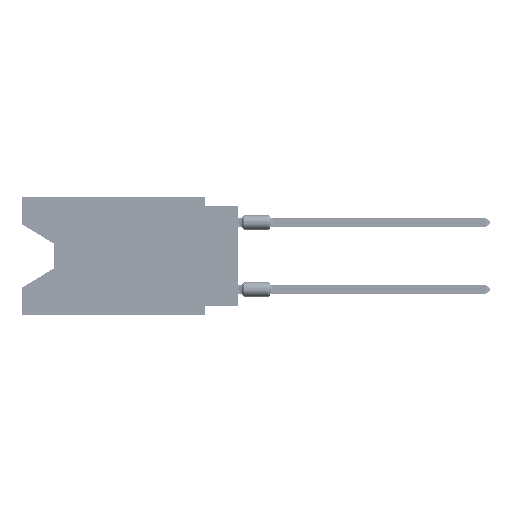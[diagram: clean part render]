
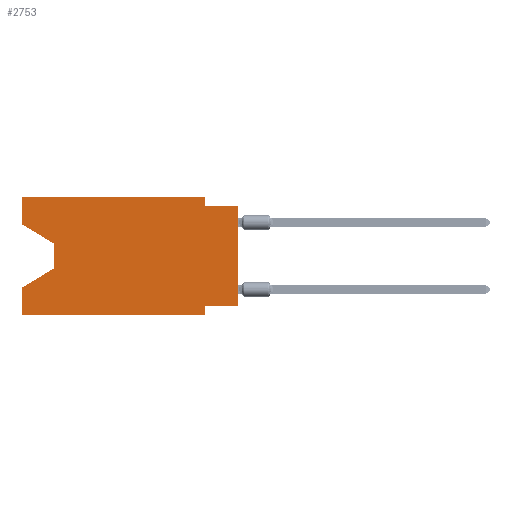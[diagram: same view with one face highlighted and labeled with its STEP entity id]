
A CAD part, left-side view. The second image highlights one B-rep face of the part: STEP entity #2753.
In plain terms, the highlighted planar face has unit normal (-1, 0, 0).
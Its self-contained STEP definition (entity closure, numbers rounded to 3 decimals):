
#519 = LINE ( 'NONE', #11945, #1159 ) ;
#1133 = VERTEX_POINT ( 'NONE', #64402 ) ;
#1159 = VECTOR ( 'NONE', #6578, 1000. ) ;
#1342 = CARTESIAN_POINT ( 'NONE',  ( 0., 2.54, -8.89 ) ) ;
#1442 = CARTESIAN_POINT ( 'NONE',  ( 0., 16.383, -2.038 ) ) ;
#2239 = CARTESIAN_POINT ( 'NONE',  ( 0., 0., -8.255 ) ) ;
#2268 = ORIENTED_EDGE ( 'NONE', *, *, #3347, .T. ) ;
#2678 = CARTESIAN_POINT ( 'NONE',  ( 0., 2.54, 0. ) ) ;
#2753 = ADVANCED_FACE ( 'NONE', ( #69702 ), #36085, .F. ) ;
#3181 = CARTESIAN_POINT ( 'NONE',  ( 0., 2.54, 0. ) ) ;
#3347 = EDGE_CURVE ( 'NONE', #59369, #17152, #27628, .T. ) ;
#3630 = VERTEX_POINT ( 'NONE', #37940 ) ;
#3878 = CARTESIAN_POINT ( 'NONE',  ( 0., 16.383, 0. ) ) ;
#5182 = LINE ( 'NONE', #21991, #12365 ) ;
#5414 = EDGE_CURVE ( 'NONE', #59369, #1133, #24259, .T. ) ;
#6153 = CARTESIAN_POINT ( 'NONE',  ( 0., 0., 0. ) ) ;
#6578 = DIRECTION ( 'NONE',  ( 0., 0., 1. ) ) ;
#7423 = EDGE_CURVE ( 'NONE', #66414, #23507, #519, .T. ) ;
#8604 = ORIENTED_EDGE ( 'NONE', *, *, #28505, .F. ) ;
#8890 = VECTOR ( 'NONE', #50507, 1000. ) ;
#11186 = VERTEX_POINT ( 'NONE', #29836 ) ;
#11945 = CARTESIAN_POINT ( 'NONE',  ( 0., 16.383, 0. ) ) ;
#12365 = VECTOR ( 'NONE', #44164, 1000. ) ;
#13409 = DIRECTION ( 'NONE',  ( 0., 0., -1. ) ) ;
#13737 = CARTESIAN_POINT ( 'NONE',  ( 0., 16.383, 0. ) ) ;
#13738 = CARTESIAN_POINT ( 'NONE',  ( 0., 16.383, -8.89 ) ) ;
#14164 = LINE ( 'NONE', #68916, #43706 ) ;
#15554 = VERTEX_POINT ( 'NONE', #50233 ) ;
#17152 = VERTEX_POINT ( 'NONE', #18348 ) ;
#17781 = DIRECTION ( 'NONE',  ( 0., 0., -1. ) ) ;
#18108 = ORIENTED_EDGE ( 'NONE', *, *, #29094, .F. ) ;
#18138 = LINE ( 'NONE', #1342, #26150 ) ;
#18348 = CARTESIAN_POINT ( 'NONE',  ( 0., 0., -0.635 ) ) ;
#18890 = CARTESIAN_POINT ( 'NONE',  ( 0., 0., -8.255 ) ) ;
#19548 = ORIENTED_EDGE ( 'NONE', *, *, #32908, .F. ) ;
#20295 = DIRECTION ( 'NONE',  ( 0., 0., -1. ) ) ;
#20742 = ORIENTED_EDGE ( 'NONE', *, *, #32326, .T. ) ;
#21483 = CARTESIAN_POINT ( 'NONE',  ( 0., 13.97, -5.385 ) ) ;
#21991 = CARTESIAN_POINT ( 'NONE',  ( 0., 0., -0.635 ) ) ;
#23507 = VERTEX_POINT ( 'NONE', #62179 ) ;
#23662 = EDGE_CURVE ( 'NONE', #39236, #63906, #57859, .T. ) ;
#24259 = LINE ( 'NONE', #18890, #60516 ) ;
#25183 = ORIENTED_EDGE ( 'NONE', *, *, #33710, .T. ) ;
#25686 = DIRECTION ( 'NONE',  ( 1., 0., 0. ) ) ;
#26150 = VECTOR ( 'NONE', #17781, 1000. ) ;
#26580 = ORIENTED_EDGE ( 'NONE', *, *, #63363, .T. ) ;
#26687 = ORIENTED_EDGE ( 'NONE', *, *, #5414, .F. ) ;
#27628 = LINE ( 'NONE', #6153, #8890 ) ;
#28505 = EDGE_CURVE ( 'NONE', #11186, #17152, #5182, .T. ) ;
#29094 = EDGE_CURVE ( 'NONE', #1133, #15554, #18138, .T. ) ;
#29836 = CARTESIAN_POINT ( 'NONE',  ( 0., 2.54, -0.635 ) ) ;
#32326 = EDGE_CURVE ( 'NONE', #63906, #23507, #66678, .T. ) ;
#32908 = EDGE_CURVE ( 'NONE', #65284, #11186, #51334, .T. ) ;
#33710 = EDGE_CURVE ( 'NONE', #46148, #39236, #67631, .T. ) ;
#35056 = CARTESIAN_POINT ( 'NONE',  ( 0., 16.383, -8.89 ) ) ;
#36085 = PLANE ( 'NONE',  #37398 ) ;
#37108 = CARTESIAN_POINT ( 'NONE',  ( 0., 13.97, -3.505 ) ) ;
#37398 = AXIS2_PLACEMENT_3D ( 'NONE', #3878, #25686, #47519 ) ;
#37940 = CARTESIAN_POINT ( 'NONE',  ( 0., 16.383, 0. ) ) ;
#38931 = ORIENTED_EDGE ( 'NONE', *, *, #56579, .F. ) ;
#39006 = DIRECTION ( 'NONE',  ( 0., -0.855, -0.519 ) ) ;
#39021 = VECTOR ( 'NONE', #61651, 1000. ) ;
#39236 = VERTEX_POINT ( 'NONE', #61716 ) ;
#39835 = CARTESIAN_POINT ( 'NONE',  ( 0., 13.97, -5.385 ) ) ;
#40435 = VECTOR ( 'NONE', #58782, 1000. ) ;
#41642 = LINE ( 'NONE', #13738, #40435 ) ;
#41718 = DIRECTION ( 'NONE',  ( 0., 0., 1. ) ) ;
#42177 = VECTOR ( 'NONE', #62758, 1000. ) ;
#43444 = CARTESIAN_POINT ( 'NONE',  ( 0., 16.383, -2.038 ) ) ;
#43706 = VECTOR ( 'NONE', #41718, 1000. ) ;
#44164 = DIRECTION ( 'NONE',  ( 0., -1., 0. ) ) ;
#46148 = VERTEX_POINT ( 'NONE', #43444 ) ;
#47519 = DIRECTION ( 'NONE',  ( 0., 0., -1. ) ) ;
#48758 = ORIENTED_EDGE ( 'NONE', *, *, #7423, .F. ) ;
#50233 = CARTESIAN_POINT ( 'NONE',  ( 0., 2.54, -8.89 ) ) ;
#50507 = DIRECTION ( 'NONE',  ( 0., 0., 1. ) ) ;
#51334 = LINE ( 'NONE', #2678, #59666 ) ;
#54314 = EDGE_LOOP ( 'NONE', ( #25183, #67473, #20742, #48758, #26580, #18108, #26687, #2268, #8604, #19548, #38931, #62961 ) ) ;
#56579 = EDGE_CURVE ( 'NONE', #3630, #65284, #57383, .T. ) ;
#57383 = LINE ( 'NONE', #13737, #42177 ) ;
#57514 = DIRECTION ( 'NONE',  ( 0., 1., 0. ) ) ;
#57859 = LINE ( 'NONE', #37108, #60787 ) ;
#58782 = DIRECTION ( 'NONE',  ( 0., -1., 0. ) ) ;
#59369 = VERTEX_POINT ( 'NONE', #2239 ) ;
#59666 = VECTOR ( 'NONE', #13409, 1000. ) ;
#60516 = VECTOR ( 'NONE', #57514, 1000. ) ;
#60787 = VECTOR ( 'NONE', #20295, 1000. ) ;
#61651 = DIRECTION ( 'NONE',  ( 0., 0.855, -0.519 ) ) ;
#61716 = CARTESIAN_POINT ( 'NONE',  ( 0., 13.97, -3.505 ) ) ;
#61726 = EDGE_CURVE ( 'NONE', #46148, #3630, #14164, .T. ) ;
#62179 = CARTESIAN_POINT ( 'NONE',  ( 0., 16.383, -6.852 ) ) ;
#62758 = DIRECTION ( 'NONE',  ( 0., -1., 0. ) ) ;
#62961 = ORIENTED_EDGE ( 'NONE', *, *, #61726, .F. ) ;
#63363 = EDGE_CURVE ( 'NONE', #66414, #15554, #41642, .T. ) ;
#63906 = VERTEX_POINT ( 'NONE', #21483 ) ;
#64402 = CARTESIAN_POINT ( 'NONE',  ( 0., 2.54, -8.255 ) ) ;
#65284 = VERTEX_POINT ( 'NONE', #3181 ) ;
#66414 = VERTEX_POINT ( 'NONE', #35056 ) ;
#66613 = VECTOR ( 'NONE', #39006, 1000. ) ;
#66678 = LINE ( 'NONE', #39835, #39021 ) ;
#67473 = ORIENTED_EDGE ( 'NONE', *, *, #23662, .T. ) ;
#67631 = LINE ( 'NONE', #1442, #66613 ) ;
#68916 = CARTESIAN_POINT ( 'NONE',  ( 0., 16.383, 0. ) ) ;
#69702 = FACE_OUTER_BOUND ( 'NONE', #54314, .T. ) ;
